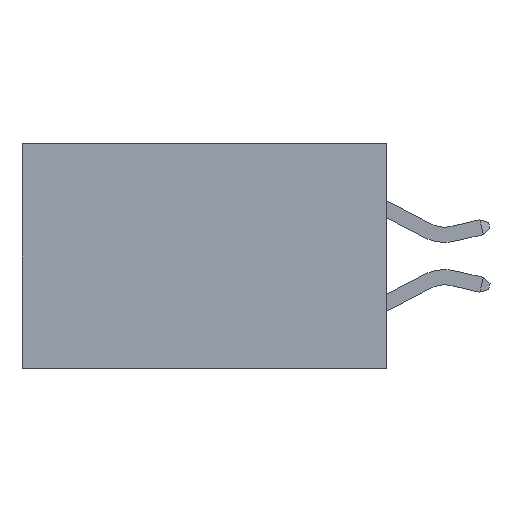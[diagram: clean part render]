
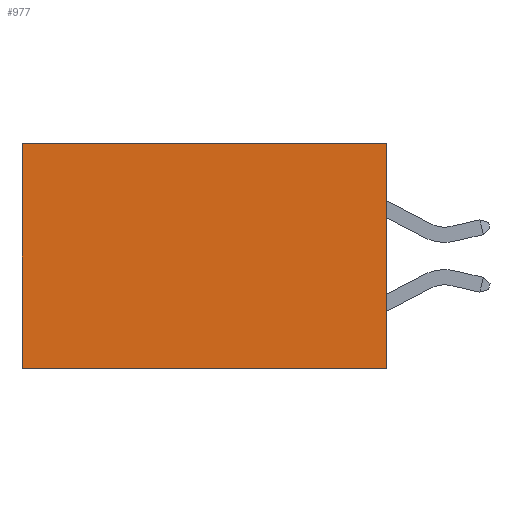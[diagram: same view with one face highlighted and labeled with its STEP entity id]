
A CAD part, left-side view. The second image highlights one B-rep face of the part: STEP entity #977.
In plain terms, the highlighted planar face has unit normal (-1, 0, 0).
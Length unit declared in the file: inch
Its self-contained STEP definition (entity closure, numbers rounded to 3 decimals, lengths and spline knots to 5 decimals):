
#244 = EDGE_CURVE ( 'NONE', #2616, #7194, #8929, .T. ) ;
#567 = EDGE_CURVE ( 'NONE', #9838, #2616, #9501, .T. ) ;
#669 = VERTEX_POINT ( 'NONE', #1830 ) ;
#872 = ORIENTED_EDGE ( 'NONE', *, *, #2841, .T. ) ;
#977 = ADVANCED_FACE ( 'NONE', ( #10690 ), #7001, .F. ) ;
#979 = VECTOR ( 'NONE', #7265, 39.37008 ) ;
#1807 = ORIENTED_EDGE ( 'NONE', *, *, #9815, .T. ) ;
#1830 = CARTESIAN_POINT ( 'NONE',  ( 0.2615, 0.6, 0. ) ) ;
#2568 = VECTOR ( 'NONE', #4573, 39.37008 ) ;
#2616 = VERTEX_POINT ( 'NONE', #7728 ) ;
#2841 = EDGE_CURVE ( 'NONE', #9838, #669, #4060, .T. ) ;
#3986 = VECTOR ( 'NONE', #9869, 39.37008 ) ;
#4060 = LINE ( 'NONE', #7136, #979 ) ;
#4100 = AXIS2_PLACEMENT_3D ( 'NONE', #10315, #10257, #6188 ) ;
#4336 = VECTOR ( 'NONE', #6972, 39.37008 ) ;
#4573 = DIRECTION ( 'NONE',  ( 0., 0., -1. ) ) ;
#5016 = CARTESIAN_POINT ( 'NONE',  ( 0.2615, 0., -0.37 ) ) ;
#5245 = ORIENTED_EDGE ( 'NONE', *, *, #567, .F. ) ;
#5918 = CARTESIAN_POINT ( 'NONE',  ( 0.2615, 0.6, -0.37 ) ) ;
#6188 = DIRECTION ( 'NONE',  ( 0., 0., -1. ) ) ;
#6337 = EDGE_LOOP ( 'NONE', ( #1807, #9887, #5245, #872 ) ) ;
#6503 = LINE ( 'NONE', #9874, #3986 ) ;
#6972 = DIRECTION ( 'NONE',  ( 0., 1., 0. ) ) ;
#7001 = PLANE ( 'NONE',  #4100 ) ;
#7136 = CARTESIAN_POINT ( 'NONE',  ( 0.2615, 0., 0. ) ) ;
#7194 = VERTEX_POINT ( 'NONE', #5918 ) ;
#7265 = DIRECTION ( 'NONE',  ( 0., 1., 0. ) ) ;
#7728 = CARTESIAN_POINT ( 'NONE',  ( 0.2615, 0., -0.37 ) ) ;
#8929 = LINE ( 'NONE', #5016, #4336 ) ;
#9501 = LINE ( 'NONE', #10126, #2568 ) ;
#9623 = CARTESIAN_POINT ( 'NONE',  ( 0.2615, 0., 0. ) ) ;
#9815 = EDGE_CURVE ( 'NONE', #669, #7194, #6503, .T. ) ;
#9838 = VERTEX_POINT ( 'NONE', #9623 ) ;
#9869 = DIRECTION ( 'NONE',  ( 0., 0., -1. ) ) ;
#9874 = CARTESIAN_POINT ( 'NONE',  ( 0.2615, 0.6, -0.37 ) ) ;
#9887 = ORIENTED_EDGE ( 'NONE', *, *, #244, .F. ) ;
#10126 = CARTESIAN_POINT ( 'NONE',  ( 0.2615, 0., -0.37 ) ) ;
#10257 = DIRECTION ( 'NONE',  ( 1., 0., 0. ) ) ;
#10315 = CARTESIAN_POINT ( 'NONE',  ( 0.2615, 0., -0.37 ) ) ;
#10690 = FACE_OUTER_BOUND ( 'NONE', #6337, .T. ) ;
